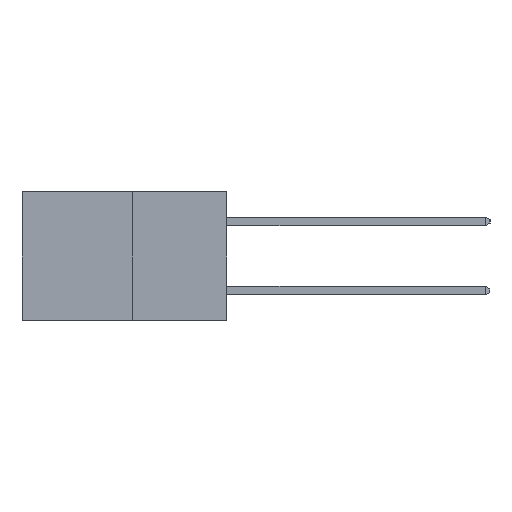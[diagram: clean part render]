
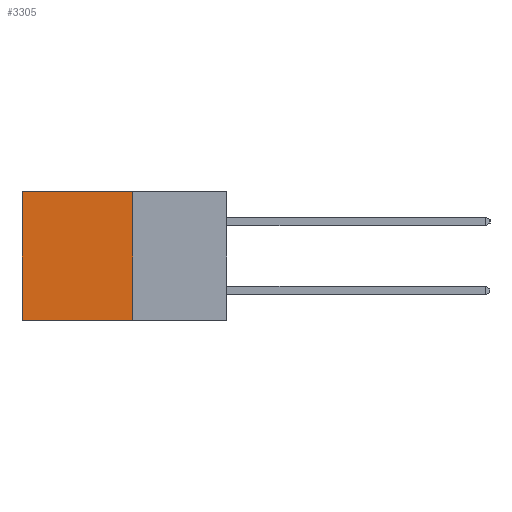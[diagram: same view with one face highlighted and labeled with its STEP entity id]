
A CAD part, left-side view. The second image highlights one B-rep face of the part: STEP entity #3305.
In plain terms, the highlighted planar face has unit normal (-1, 0, 0).
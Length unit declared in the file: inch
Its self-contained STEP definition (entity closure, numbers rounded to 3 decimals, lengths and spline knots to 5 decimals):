
#63 = VERTEX_POINT ( 'NONE', #19523 ) ;
#646 = DIRECTION ( 'NONE',  ( 0., 1., 0. ) ) ;
#1013 = VERTEX_POINT ( 'NONE', #16183 ) ;
#1784 = LINE ( 'NONE', #21282, #15087 ) ;
#1888 = DIRECTION ( 'NONE',  ( 0., 0., -1. ) ) ;
#2025 = DIRECTION ( 'NONE',  ( 1., 0., 0. ) ) ;
#2130 = PLANE ( 'NONE',  #12585 ) ;
#2221 = VERTEX_POINT ( 'NONE', #16004 ) ;
#2388 = ORIENTED_EDGE ( 'NONE', *, *, #14090, .F. ) ;
#3305 = ADVANCED_FACE ( 'NONE', ( #13762 ), #2130, .F. ) ;
#4176 = CARTESIAN_POINT ( 'NONE',  ( 0.277, 0.27, -0.37 ) ) ;
#5322 = EDGE_CURVE ( 'NONE', #63, #19286, #8761, .T. ) ;
#6067 = EDGE_LOOP ( 'NONE', ( #9879, #15800, #2388, #21585 ) ) ;
#6903 = LINE ( 'NONE', #9408, #15516 ) ;
#7892 = DIRECTION ( 'NONE',  ( 0., 0., -1. ) ) ;
#8103 = CARTESIAN_POINT ( 'NONE',  ( 0.277, 0.59, -0.37 ) ) ;
#8338 = VECTOR ( 'NONE', #12972, 39.37008 ) ;
#8761 = LINE ( 'NONE', #8103, #17356 ) ;
#9408 = CARTESIAN_POINT ( 'NONE',  ( 0.277, 0.27, -0.37 ) ) ;
#9879 = ORIENTED_EDGE ( 'NONE', *, *, #5322, .T. ) ;
#11147 = DIRECTION ( 'NONE',  ( 0., 1., 0. ) ) ;
#11265 = CARTESIAN_POINT ( 'NONE',  ( 0.277, 0.27, -0.37 ) ) ;
#12585 = AXIS2_PLACEMENT_3D ( 'NONE', #4176, #2025, #1888 ) ;
#12972 = DIRECTION ( 'NONE',  ( 0., 0., -1. ) ) ;
#13762 = FACE_OUTER_BOUND ( 'NONE', #6067, .T. ) ;
#14090 = EDGE_CURVE ( 'NONE', #1013, #2221, #21863, .T. ) ;
#14378 = CARTESIAN_POINT ( 'NONE',  ( 0.277, 0.59, -0.37 ) ) ;
#15087 = VECTOR ( 'NONE', #646, 39.37008 ) ;
#15516 = VECTOR ( 'NONE', #11147, 39.37008 ) ;
#15800 = ORIENTED_EDGE ( 'NONE', *, *, #20605, .F. ) ;
#16004 = CARTESIAN_POINT ( 'NONE',  ( 0.277, 0.27, -0.37 ) ) ;
#16183 = CARTESIAN_POINT ( 'NONE',  ( 0.277, 0.27, 0. ) ) ;
#17356 = VECTOR ( 'NONE', #7892, 39.37008 ) ;
#17484 = EDGE_CURVE ( 'NONE', #1013, #63, #1784, .T. ) ;
#19286 = VERTEX_POINT ( 'NONE', #14378 ) ;
#19523 = CARTESIAN_POINT ( 'NONE',  ( 0.277, 0.59, 0. ) ) ;
#20605 = EDGE_CURVE ( 'NONE', #2221, #19286, #6903, .T. ) ;
#21282 = CARTESIAN_POINT ( 'NONE',  ( 0.277, 0.27, 0. ) ) ;
#21585 = ORIENTED_EDGE ( 'NONE', *, *, #17484, .T. ) ;
#21863 = LINE ( 'NONE', #11265, #8338 ) ;
